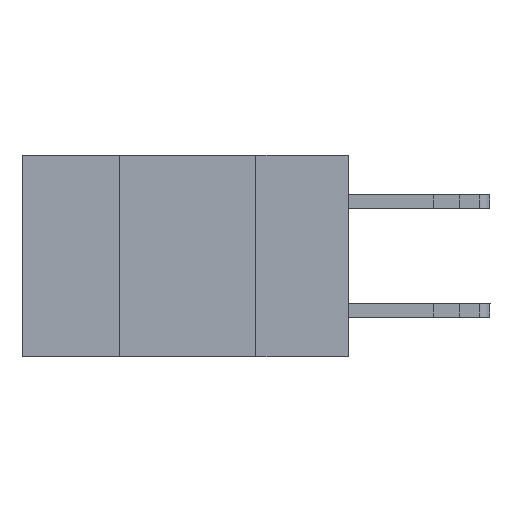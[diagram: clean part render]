
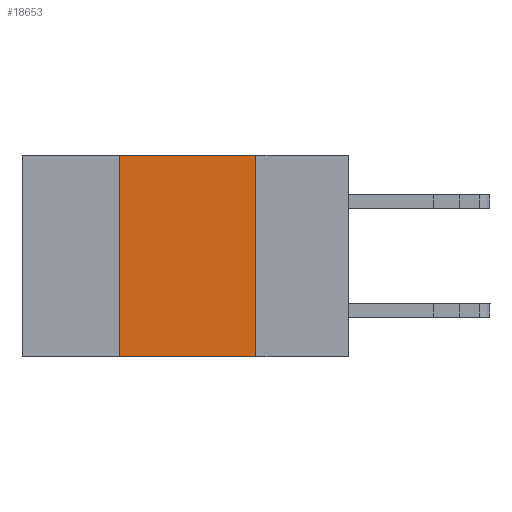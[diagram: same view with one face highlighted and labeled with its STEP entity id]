
A CAD part, left-side view. The second image highlights one B-rep face of the part: STEP entity #18653.
In plain terms, the highlighted planar face has unit normal (-1, 0, 0).
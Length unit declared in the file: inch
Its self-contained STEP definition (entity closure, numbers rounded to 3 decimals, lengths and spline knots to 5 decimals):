
#1025 = VECTOR ( 'NONE', #3177, 39.37008 ) ;
#1226 = ORIENTED_EDGE ( 'NONE', *, *, #3616, .F. ) ;
#1306 = EDGE_CURVE ( 'NONE', #4441, #14468, #18405, .T. ) ;
#2042 = CARTESIAN_POINT ( 'NONE',  ( 0., 0.17, 0. ) ) ;
#2044 = DIRECTION ( 'NONE',  ( 0., 0., 1. ) ) ;
#2186 = CARTESIAN_POINT ( 'NONE',  ( 0., 0.42, -0.37 ) ) ;
#2235 = AXIS2_PLACEMENT_3D ( 'NONE', #7174, #18787, #10091 ) ;
#3177 = DIRECTION ( 'NONE',  ( 0., -1., 0. ) ) ;
#3616 = EDGE_CURVE ( 'NONE', #8793, #15330, #15883, .T. ) ;
#4000 = CARTESIAN_POINT ( 'NONE',  ( 0., 0.17, -0.37 ) ) ;
#4296 = LINE ( 'NONE', #4380, #8679 ) ;
#4380 = CARTESIAN_POINT ( 'NONE',  ( 0., 0.6, 0. ) ) ;
#4441 = VERTEX_POINT ( 'NONE', #4854 ) ;
#4854 = CARTESIAN_POINT ( 'NONE',  ( 0., 0.42, -0.37 ) ) ;
#5052 = LINE ( 'NONE', #7619, #1025 ) ;
#6273 = CARTESIAN_POINT ( 'NONE',  ( 0., 0.17, -0.37 ) ) ;
#6386 = DIRECTION ( 'NONE',  ( 0., 0., -1. ) ) ;
#7174 = CARTESIAN_POINT ( 'NONE',  ( 0., 0.6, 0. ) ) ;
#7619 = CARTESIAN_POINT ( 'NONE',  ( 0., 0.6, -0.37 ) ) ;
#8679 = VECTOR ( 'NONE', #14662, 39.37008 ) ;
#8793 = VERTEX_POINT ( 'NONE', #2042 ) ;
#8881 = EDGE_LOOP ( 'NONE', ( #1226, #10984, #16021, #16980 ) ) ;
#10091 = DIRECTION ( 'NONE',  ( 0., 0., -1. ) ) ;
#10984 = ORIENTED_EDGE ( 'NONE', *, *, #13333, .F. ) ;
#11505 = EDGE_CURVE ( 'NONE', #4441, #15330, #5052, .T. ) ;
#13333 = EDGE_CURVE ( 'NONE', #14468, #8793, #4296, .T. ) ;
#14468 = VERTEX_POINT ( 'NONE', #16826 ) ;
#14601 = VECTOR ( 'NONE', #2044, 39.37008 ) ;
#14662 = DIRECTION ( 'NONE',  ( 0., -1., 0. ) ) ;
#15330 = VERTEX_POINT ( 'NONE', #4000 ) ;
#15431 = VECTOR ( 'NONE', #6386, 39.37008 ) ;
#15883 = LINE ( 'NONE', #6273, #15431 ) ;
#15917 = PLANE ( 'NONE',  #2235 ) ;
#16021 = ORIENTED_EDGE ( 'NONE', *, *, #1306, .F. ) ;
#16493 = FACE_OUTER_BOUND ( 'NONE', #8881, .T. ) ;
#16826 = CARTESIAN_POINT ( 'NONE',  ( 0., 0.42, 0. ) ) ;
#16980 = ORIENTED_EDGE ( 'NONE', *, *, #11505, .T. ) ;
#18405 = LINE ( 'NONE', #2186, #14601 ) ;
#18653 = ADVANCED_FACE ( 'NONE', ( #16493 ), #15917, .F. ) ;
#18787 = DIRECTION ( 'NONE',  ( 1., 0., 0. ) ) ;
